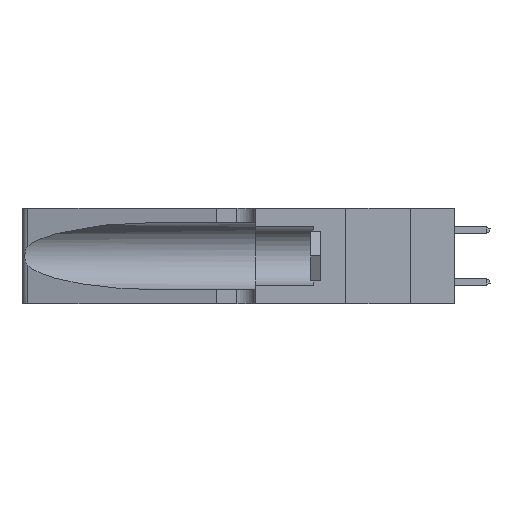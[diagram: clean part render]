
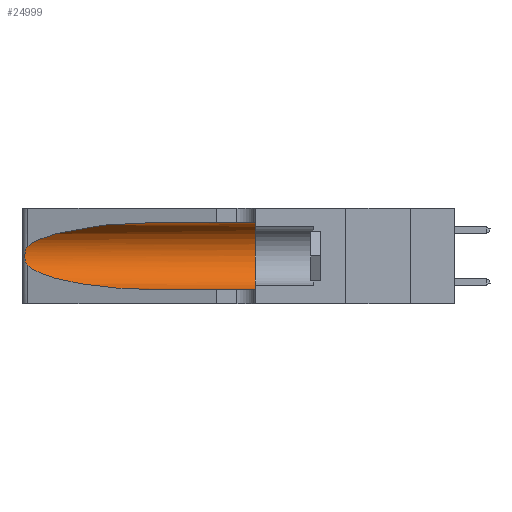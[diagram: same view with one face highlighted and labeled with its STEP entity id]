
A CAD part, left-side view. The second image highlights one B-rep face of the part: STEP entity #24999.
In plain terms, the highlighted cylindrical face has radius 3.308 mm (diameter 6.617 mm), a partial arc.
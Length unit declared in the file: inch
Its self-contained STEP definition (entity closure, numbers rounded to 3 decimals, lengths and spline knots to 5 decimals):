
#131 = ORIENTED_EDGE ( 'NONE', *, *, #17818, .T. ) ;
#930 = EDGE_CURVE ( 'NONE', #25681, #18180, #18440, .T. ) ;
#1212 = CARTESIAN_POINT ( 'NONE',  ( 0.25487, 1.22718, 0.14631 ) ) ;
#1505 = CARTESIAN_POINT ( 'NONE',  ( 0.25854, 1.2359, 0.20912 ) ) ;
#2083 = EDGE_LOOP ( 'NONE', ( #30759, #131, #15992, #23036, #5852, #17378 ) ) ;
#3581 = EDGE_CURVE ( 'NONE', #43893, #21382, #35221, .T. ) ;
#5093 = CARTESIAN_POINT ( 'NONE',  ( 0.25639, 1.23184, 0.21858 ) ) ;
#5852 = ORIENTED_EDGE ( 'NONE', *, *, #32990, .F. ) ;
#6169 = CARTESIAN_POINT ( 'NONE',  ( 0.1305, 1.61858, 0.185 ) ) ;
#6421 = AXIS2_PLACEMENT_3D ( 'NONE', #12625, #19478, #12478 ) ;
#8304 = CARTESIAN_POINT ( 'NONE',  ( 0.26075, 1.23896, 0.178 ) ) ;
#8455 = CARTESIAN_POINT ( 'NONE',  ( 0.26018, 1.23835, 0.19895 ) ) ;
#9470 = CARTESIAN_POINT ( 'NONE',  ( 0.1305, 1.61858, 0.05475 ) ) ;
#12478 = DIRECTION ( 'NONE',  ( 0., 0., 1. ) ) ;
#12625 = CARTESIAN_POINT ( 'NONE',  ( 0.1305, 0.35, 0.185 ) ) ;
#12699 = EDGE_CURVE ( 'NONE', #42637, #25681, #40369, .T. ) ;
#15131 = CARTESIAN_POINT ( 'NONE',  ( 0.25487, 1.22718, 0.22369 ) ) ;
#15992 = ORIENTED_EDGE ( 'NONE', *, *, #12699, .T. ) ;
#16259 = CARTESIAN_POINT ( 'NONE',  ( 0.1305, 0.35, 0.31525 ) ) ;
#17378 = ORIENTED_EDGE ( 'NONE', *, *, #3581, .F. ) ;
#17461 = VERTEX_POINT ( 'NONE', #37459 ) ;
#17818 = EDGE_CURVE ( 'NONE', #17461, #42637, #32176, .T. ) ;
#18180 = VERTEX_POINT ( 'NONE', #37706 ) ;
#18440 = LINE ( 'NONE', #9470, #34945 ) ;
#18826 = CARTESIAN_POINT ( 'NONE',  ( 0.26017, 1.23833, 0.17102 ) ) ;
#19299 = CARTESIAN_POINT ( 'NONE',  ( 0.25555, 1.22993, 0.14849 ) ) ;
#19478 = DIRECTION ( 'NONE',  ( 0., 1., 0. ) ) ;
#19791 = AXIS2_PLACEMENT_3D ( 'NONE', #6169, #37578, #44542 ) ;
#20066 = FACE_OUTER_BOUND ( 'NONE', #2083, .T. ) ;
#20998 = CARTESIAN_POINT ( 'NONE',  ( 0.25487, 1.22718, 0.22369 ) ) ;
#21264 = CARTESIAN_POINT ( 'NONE',  ( 0.25487, 1.22718, 0.14631 ) ) ;
#21382 = VERTEX_POINT ( 'NONE', #16259 ) ;
#22220 = CARTESIAN_POINT ( 'NONE',  ( 0.25789, 1.23486, 0.15765 ) ) ;
#22823 = CYLINDRICAL_SURFACE ( 'NONE', #19791, 0.13025 ) ;
#23036 = ORIENTED_EDGE ( 'NONE', *, *, #930, .T. ) ;
#23094 = DIRECTION ( 'NONE',  ( 0., -1., 0. ) ) ;
#24524 = CARTESIAN_POINT ( 'NONE',  ( 0.2373, 1.15595, 0.08982 ) ) ;
#24680 = CARTESIAN_POINT ( 'NONE',  ( 0.1305, 0.72297, 0.05475 ) ) ;
#24817 = VECTOR ( 'NONE', #39175, 39.37008 ) ;
#24999 = ADVANCED_FACE ( 'NONE', ( #20066 ), #22823, .F. ) ;
#25681 = VERTEX_POINT ( 'NONE', #44484 ) ;
#26091 = CARTESIAN_POINT ( 'NONE',  ( 0.25639, 1.23186, 0.15144 ) ) ;
#27984 =( BOUNDED_CURVE ( )  B_SPLINE_CURVE ( 3, ( #31568, #38493, #28366, #20998 ),
 .UNSPECIFIED., .F., .F. ) 
 B_SPLINE_CURVE_WITH_KNOTS ( ( 4, 4 ),
 ( 1.5708, 2.84003 ),
 .UNSPECIFIED. ) 
 CURVE ( )  GEOMETRIC_REPRESENTATION_ITEM ( )  RATIONAL_B_SPLINE_CURVE ( ( 1., 0.87, 0.87, 1. ) ) 
 REPRESENTATION_ITEM ( '' )  );
#28366 = CARTESIAN_POINT ( 'NONE',  ( 0.2373, 1.15595, 0.28018 ) ) ;
#30759 = ORIENTED_EDGE ( 'NONE', *, *, #41838, .T. ) ;
#31568 = CARTESIAN_POINT ( 'NONE',  ( 0.1305, 0.72297, 0.31525 ) ) ;
#32176 = B_SPLINE_CURVE_WITH_KNOTS ( 'NONE', 3,
 ( #15131, #43311, #5093, #32986, #1505, #8455, #36811, #8304, #18826, #32675, #22220, #26091, #19299, #43923 ),
 .UNSPECIFIED., .F., .F.,
 ( 4, 2, 2, 2, 2, 2, 4 ),
 ( 0., 0.00027, 0.00053, 0.00107, 0.0016, 0.00187, 0.00214 ),
 .UNSPECIFIED. ) ;
#32675 = CARTESIAN_POINT ( 'NONE',  ( 0.25856, 1.23593, 0.16098 ) ) ;
#32986 = CARTESIAN_POINT ( 'NONE',  ( 0.25787, 1.23484, 0.2124 ) ) ;
#32990 = EDGE_CURVE ( 'NONE', #21382, #18180, #35026, .T. ) ;
#34945 = VECTOR ( 'NONE', #23094, 39.37008 ) ;
#35026 = CIRCLE ( 'NONE', #6421, 0.13025 ) ;
#35221 = LINE ( 'NONE', #39027, #24817 ) ;
#35390 = CARTESIAN_POINT ( 'NONE',  ( 0.18966, 0.96281, 0.05475 ) ) ;
#36811 = CARTESIAN_POINT ( 'NONE',  ( 0.26075, 1.23896, 0.19203 ) ) ;
#37459 = CARTESIAN_POINT ( 'NONE',  ( 0.25487, 1.22718, 0.22369 ) ) ;
#37578 = DIRECTION ( 'NONE',  ( 0., -1., 0. ) ) ;
#37639 = CARTESIAN_POINT ( 'NONE',  ( 0.1305, 0.72297, 0.31525 ) ) ;
#37706 = CARTESIAN_POINT ( 'NONE',  ( 0.1305, 0.35, 0.05475 ) ) ;
#38493 = CARTESIAN_POINT ( 'NONE',  ( 0.18966, 0.96281, 0.31525 ) ) ;
#39027 = CARTESIAN_POINT ( 'NONE',  ( 0.1305, 1.61858, 0.31525 ) ) ;
#39175 = DIRECTION ( 'NONE',  ( 0., -1., 0. ) ) ;
#40369 =( BOUNDED_CURVE ( )  B_SPLINE_CURVE ( 3, ( #21264, #24524, #35390, #24680 ),
 .UNSPECIFIED., .F., .T. ) 
 B_SPLINE_CURVE_WITH_KNOTS ( ( 4, 4 ),
 ( 3.44316, 4.71239 ),
 .UNSPECIFIED. ) 
 CURVE ( )  GEOMETRIC_REPRESENTATION_ITEM ( )  RATIONAL_B_SPLINE_CURVE ( ( 1., 0.87, 0.87, 1. ) ) 
 REPRESENTATION_ITEM ( '' )  );
#41838 = EDGE_CURVE ( 'NONE', #43893, #17461, #27984, .T. ) ;
#42637 = VERTEX_POINT ( 'NONE', #1212 ) ;
#43311 = CARTESIAN_POINT ( 'NONE',  ( 0.25555, 1.22994, 0.2215 ) ) ;
#43893 = VERTEX_POINT ( 'NONE', #37639 ) ;
#43923 = CARTESIAN_POINT ( 'NONE',  ( 0.25487, 1.22718, 0.14631 ) ) ;
#44484 = CARTESIAN_POINT ( 'NONE',  ( 0.1305, 0.72297, 0.05475 ) ) ;
#44542 = DIRECTION ( 'NONE',  ( 0., 0., -1. ) ) ;
